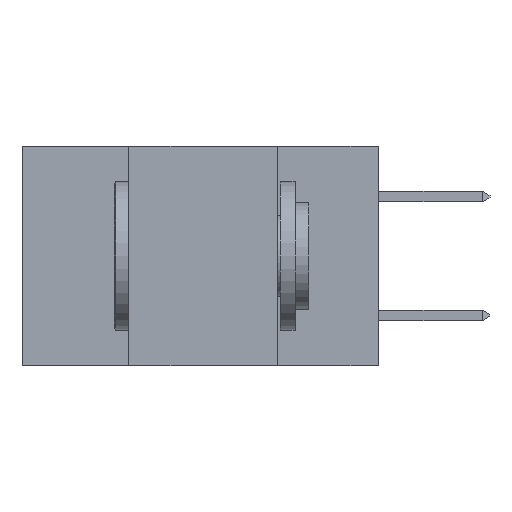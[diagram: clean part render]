
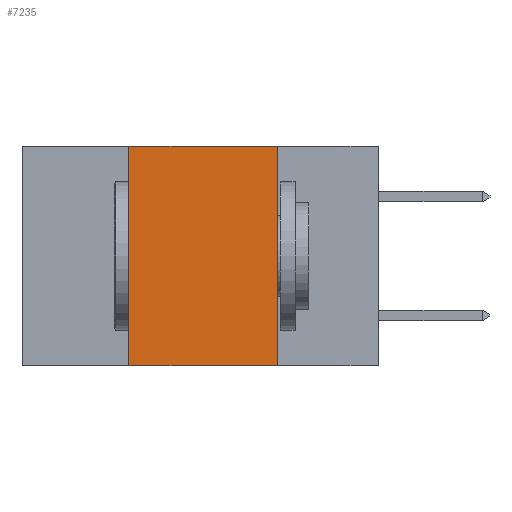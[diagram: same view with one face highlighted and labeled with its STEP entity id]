
A CAD part, left-side view. The second image highlights one B-rep face of the part: STEP entity #7235.
In plain terms, the highlighted planar face has unit normal (-1, 0, 0).
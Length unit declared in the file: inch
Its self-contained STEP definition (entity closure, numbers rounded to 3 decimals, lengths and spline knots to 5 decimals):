
#78 = CARTESIAN_POINT ( 'NONE',  ( 0., 0.17, -0.37 ) ) ;
#504 = VERTEX_POINT ( 'NONE', #8425 ) ;
#526 = CARTESIAN_POINT ( 'NONE',  ( 0., 0.6, 0. ) ) ;
#2193 = ORIENTED_EDGE ( 'NONE', *, *, #10498, .F. ) ;
#2260 = EDGE_CURVE ( 'NONE', #504, #18231, #5615, .T. ) ;
#2429 = CARTESIAN_POINT ( 'NONE',  ( 0., 0.6, 0. ) ) ;
#2704 = EDGE_CURVE ( 'NONE', #504, #22047, #5590, .T. ) ;
#3240 = ORIENTED_EDGE ( 'NONE', *, *, #2704, .F. ) ;
#4223 = DIRECTION ( 'NONE',  ( 1., 0., 0. ) ) ;
#4944 = CARTESIAN_POINT ( 'NONE',  ( 0., 0.42, 0. ) ) ;
#5590 = LINE ( 'NONE', #11065, #9932 ) ;
#5615 = LINE ( 'NONE', #6783, #14842 ) ;
#5885 = DIRECTION ( 'NONE',  ( 0., -1., 0. ) ) ;
#5961 = EDGE_CURVE ( 'NONE', #17644, #18231, #11532, .T. ) ;
#6607 = VECTOR ( 'NONE', #21298, 39.37008 ) ;
#6783 = CARTESIAN_POINT ( 'NONE',  ( 0., 0.6, -0.37 ) ) ;
#7235 = ADVANCED_FACE ( 'NONE', ( #10934 ), #22558, .F. ) ;
#8425 = CARTESIAN_POINT ( 'NONE',  ( 0., 0.42, -0.37 ) ) ;
#9626 = ORIENTED_EDGE ( 'NONE', *, *, #2260, .T. ) ;
#9932 = VECTOR ( 'NONE', #12219, 39.37008 ) ;
#10498 = EDGE_CURVE ( 'NONE', #22047, #17644, #17645, .T. ) ;
#10801 = AXIS2_PLACEMENT_3D ( 'NONE', #526, #4223, #17095 ) ;
#10934 = FACE_OUTER_BOUND ( 'NONE', #12792, .T. ) ;
#11065 = CARTESIAN_POINT ( 'NONE',  ( 0., 0.42, 0. ) ) ;
#11532 = LINE ( 'NONE', #11964, #6607 ) ;
#11964 = CARTESIAN_POINT ( 'NONE',  ( 0., 0.17, 0. ) ) ;
#12219 = DIRECTION ( 'NONE',  ( 0., 0., 1. ) ) ;
#12792 = EDGE_LOOP ( 'NONE', ( #14343, #2193, #3240, #9626 ) ) ;
#12833 = CARTESIAN_POINT ( 'NONE',  ( 0., 0.17, 0. ) ) ;
#14343 = ORIENTED_EDGE ( 'NONE', *, *, #5961, .F. ) ;
#14842 = VECTOR ( 'NONE', #5885, 39.37008 ) ;
#17095 = DIRECTION ( 'NONE',  ( 0., 0., -1. ) ) ;
#17142 = DIRECTION ( 'NONE',  ( 0., -1., 0. ) ) ;
#17644 = VERTEX_POINT ( 'NONE', #12833 ) ;
#17645 = LINE ( 'NONE', #2429, #21990 ) ;
#18231 = VERTEX_POINT ( 'NONE', #78 ) ;
#21298 = DIRECTION ( 'NONE',  ( 0., 0., -1. ) ) ;
#21990 = VECTOR ( 'NONE', #17142, 39.37008 ) ;
#22047 = VERTEX_POINT ( 'NONE', #4944 ) ;
#22558 = PLANE ( 'NONE',  #10801 ) ;
